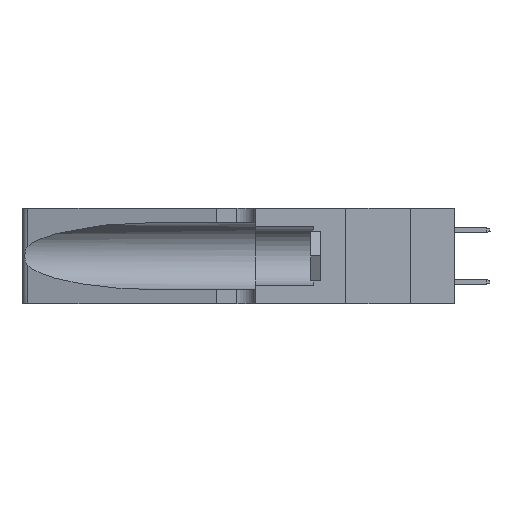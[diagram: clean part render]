
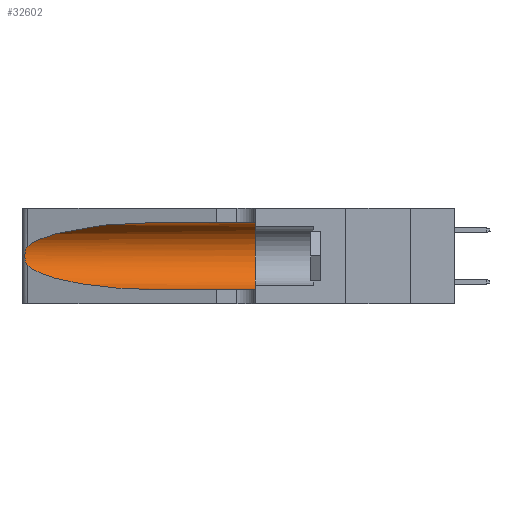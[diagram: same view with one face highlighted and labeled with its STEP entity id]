
A CAD part, left-side view. The second image highlights one B-rep face of the part: STEP entity #32602.
In plain terms, the highlighted cylindrical face has radius 3.308 mm (diameter 6.617 mm), a partial arc.
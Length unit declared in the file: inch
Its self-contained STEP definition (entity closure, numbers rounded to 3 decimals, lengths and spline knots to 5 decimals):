
#316 = CARTESIAN_POINT ( 'NONE',  ( 0.25487, 1.22718, 0.14631 ) ) ;
#318 = FACE_OUTER_BOUND ( 'NONE', #19461, .T. ) ;
#341 = VERTEX_POINT ( 'NONE', #31248 ) ;
#606 =( BOUNDED_CURVE ( )  B_SPLINE_CURVE ( 3, ( #19152, #41895, #35992, #15675 ),
 .UNSPECIFIED., .F., .T. ) 
 B_SPLINE_CURVE_WITH_KNOTS ( ( 4, 4 ),
 ( 1.5708, 2.84003 ),
 .UNSPECIFIED. ) 
 CURVE ( )  GEOMETRIC_REPRESENTATION_ITEM ( )  RATIONAL_B_SPLINE_CURVE ( ( 1., 0.87, 0.87, 1. ) ) 
 REPRESENTATION_ITEM ( '' )  );
#4022 = VECTOR ( 'NONE', #15362, 39.37008 ) ;
#4025 = DIRECTION ( 'NONE',  ( 0., -1., 0. ) ) ;
#4127 = ORIENTED_EDGE ( 'NONE', *, *, #12148, .F. ) ;
#4589 = CARTESIAN_POINT ( 'NONE',  ( 0.1305, 0.35, 0.05475 ) ) ;
#7733 = CARTESIAN_POINT ( 'NONE',  ( 0.25555, 1.22993, 0.14849 ) ) ;
#8458 = VERTEX_POINT ( 'NONE', #37341 ) ;
#9741 = VERTEX_POINT ( 'NONE', #20332 ) ;
#11194 = ORIENTED_EDGE ( 'NONE', *, *, #35981, .T. ) ;
#11450 = CARTESIAN_POINT ( 'NONE',  ( 0.26018, 1.23835, 0.19895 ) ) ;
#11556 = VECTOR ( 'NONE', #34346, 39.37008 ) ;
#12097 = VERTEX_POINT ( 'NONE', #4589 ) ;
#12148 = EDGE_CURVE ( 'NONE', #24596, #12097, #34664, .T. ) ;
#12873 = B_SPLINE_CURVE_WITH_KNOTS ( 'NONE', 3,
 ( #41142, #24992, #41362, #25204, #17768, #11450, #24761, #31089, #40921, #28244, #37889, #38536, #7733, #21038 ),
 .UNSPECIFIED., .F., .F.,
 ( 4, 2, 2, 2, 2, 2, 4 ),
 ( 0., 0.00027, 0.00053, 0.00107, 0.0016, 0.00187, 0.00214 ),
 .UNSPECIFIED. ) ;
#13423 = CYLINDRICAL_SURFACE ( 'NONE', #38170, 0.13025 ) ;
#13998 =( BOUNDED_CURVE ( )  B_SPLINE_CURVE ( 3, ( #16631, #29951, #16844, #30166 ),
 .UNSPECIFIED., .F., .T. ) 
 B_SPLINE_CURVE_WITH_KNOTS ( ( 4, 4 ),
 ( 3.44316, 4.71239 ),
 .UNSPECIFIED. ) 
 CURVE ( )  GEOMETRIC_REPRESENTATION_ITEM ( )  RATIONAL_B_SPLINE_CURVE ( ( 1., 0.87, 0.87, 1. ) ) 
 REPRESENTATION_ITEM ( '' )  );
#15362 = DIRECTION ( 'NONE',  ( 0., -1., 0. ) ) ;
#15675 = CARTESIAN_POINT ( 'NONE',  ( 0.25487, 1.22718, 0.22369 ) ) ;
#16631 = CARTESIAN_POINT ( 'NONE',  ( 0.25487, 1.22718, 0.14631 ) ) ;
#16844 = CARTESIAN_POINT ( 'NONE',  ( 0.18966, 0.96281, 0.05475 ) ) ;
#17498 = CARTESIAN_POINT ( 'NONE',  ( 0.1305, 1.61858, 0.31525 ) ) ;
#17768 = CARTESIAN_POINT ( 'NONE',  ( 0.25854, 1.2359, 0.20912 ) ) ;
#18555 = CARTESIAN_POINT ( 'NONE',  ( 0.1305, 0.35, 0.185 ) ) ;
#19152 = CARTESIAN_POINT ( 'NONE',  ( 0.1305, 0.72297, 0.31525 ) ) ;
#19461 = EDGE_LOOP ( 'NONE', ( #11194, #34418, #38509, #37680, #4127, #34525 ) ) ;
#20332 = CARTESIAN_POINT ( 'NONE',  ( 0.1305, 0.72297, 0.05475 ) ) ;
#21038 = CARTESIAN_POINT ( 'NONE',  ( 0.25487, 1.22718, 0.14631 ) ) ;
#21384 = AXIS2_PLACEMENT_3D ( 'NONE', #18555, #27522, #38456 ) ;
#24596 = VERTEX_POINT ( 'NONE', #25723 ) ;
#24761 = CARTESIAN_POINT ( 'NONE',  ( 0.26075, 1.23896, 0.19203 ) ) ;
#24992 = CARTESIAN_POINT ( 'NONE',  ( 0.25555, 1.22994, 0.2215 ) ) ;
#25204 = CARTESIAN_POINT ( 'NONE',  ( 0.25787, 1.23484, 0.2124 ) ) ;
#25723 = CARTESIAN_POINT ( 'NONE',  ( 0.1305, 0.35, 0.31525 ) ) ;
#27253 = VERTEX_POINT ( 'NONE', #316 ) ;
#27522 = DIRECTION ( 'NONE',  ( 0., 1., 0. ) ) ;
#28244 = CARTESIAN_POINT ( 'NONE',  ( 0.25856, 1.23593, 0.16098 ) ) ;
#28460 = CARTESIAN_POINT ( 'NONE',  ( 0.1305, 1.61858, 0.05475 ) ) ;
#29951 = CARTESIAN_POINT ( 'NONE',  ( 0.2373, 1.15595, 0.08982 ) ) ;
#30166 = CARTESIAN_POINT ( 'NONE',  ( 0.1305, 0.72297, 0.05475 ) ) ;
#30224 = CARTESIAN_POINT ( 'NONE',  ( 0.1305, 1.61858, 0.185 ) ) ;
#30505 = EDGE_CURVE ( 'NONE', #8458, #24596, #34130, .T. ) ;
#31089 = CARTESIAN_POINT ( 'NONE',  ( 0.26075, 1.23896, 0.178 ) ) ;
#31248 = CARTESIAN_POINT ( 'NONE',  ( 0.25487, 1.22718, 0.22369 ) ) ;
#32602 = ADVANCED_FACE ( 'NONE', ( #318 ), #13423, .F. ) ;
#32755 = EDGE_CURVE ( 'NONE', #341, #27253, #12873, .T. ) ;
#34130 = LINE ( 'NONE', #17498, #11556 ) ;
#34346 = DIRECTION ( 'NONE',  ( 0., -1., 0. ) ) ;
#34418 = ORIENTED_EDGE ( 'NONE', *, *, #32755, .T. ) ;
#34525 = ORIENTED_EDGE ( 'NONE', *, *, #30505, .F. ) ;
#34664 = CIRCLE ( 'NONE', #21384, 0.13025 ) ;
#35981 = EDGE_CURVE ( 'NONE', #8458, #341, #606, .T. ) ;
#35992 = CARTESIAN_POINT ( 'NONE',  ( 0.2373, 1.15595, 0.28018 ) ) ;
#37341 = CARTESIAN_POINT ( 'NONE',  ( 0.1305, 0.72297, 0.31525 ) ) ;
#37680 = ORIENTED_EDGE ( 'NONE', *, *, #38210, .T. ) ;
#37889 = CARTESIAN_POINT ( 'NONE',  ( 0.25789, 1.23486, 0.15765 ) ) ;
#38170 = AXIS2_PLACEMENT_3D ( 'NONE', #30224, #4025, #40488 ) ;
#38210 = EDGE_CURVE ( 'NONE', #9741, #12097, #39382, .T. ) ;
#38381 = EDGE_CURVE ( 'NONE', #27253, #9741, #13998, .T. ) ;
#38456 = DIRECTION ( 'NONE',  ( 0., 0., 1. ) ) ;
#38509 = ORIENTED_EDGE ( 'NONE', *, *, #38381, .T. ) ;
#38536 = CARTESIAN_POINT ( 'NONE',  ( 0.25639, 1.23186, 0.15144 ) ) ;
#39382 = LINE ( 'NONE', #28460, #4022 ) ;
#40488 = DIRECTION ( 'NONE',  ( 0., 0., -1. ) ) ;
#40921 = CARTESIAN_POINT ( 'NONE',  ( 0.26017, 1.23833, 0.17102 ) ) ;
#41142 = CARTESIAN_POINT ( 'NONE',  ( 0.25487, 1.22718, 0.22369 ) ) ;
#41362 = CARTESIAN_POINT ( 'NONE',  ( 0.25639, 1.23184, 0.21858 ) ) ;
#41895 = CARTESIAN_POINT ( 'NONE',  ( 0.18966, 0.96281, 0.31525 ) ) ;
